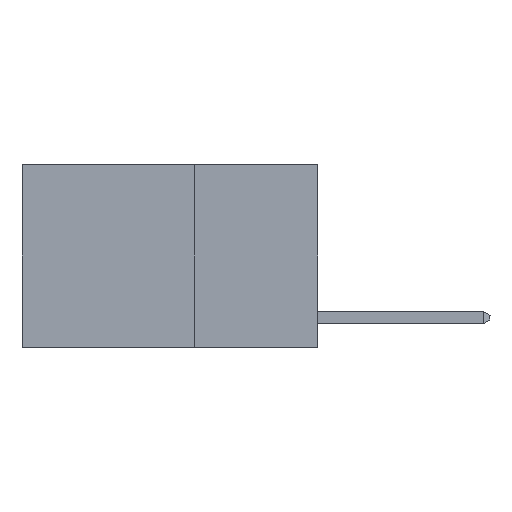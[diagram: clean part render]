
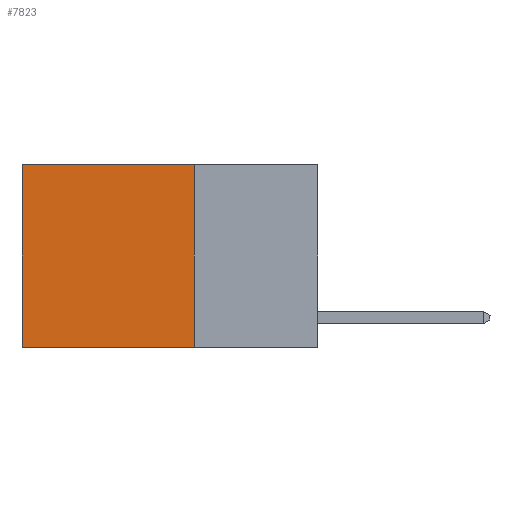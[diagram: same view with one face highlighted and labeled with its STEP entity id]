
A CAD part, left-side view. The second image highlights one B-rep face of the part: STEP entity #7823.
In plain terms, the highlighted planar face has unit normal (-1, 0, 0).
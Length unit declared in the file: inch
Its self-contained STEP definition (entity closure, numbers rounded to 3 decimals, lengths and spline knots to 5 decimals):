
#1244 = LINE ( 'NONE', #2165, #11962 ) ;
#1682 = FACE_OUTER_BOUND ( 'NONE', #6135, .T. ) ;
#2165 = CARTESIAN_POINT ( 'NONE',  ( 0.2625, 0.6, 0. ) ) ;
#3813 = DIRECTION ( 'NONE',  ( 0., 1., 0. ) ) ;
#4150 = CARTESIAN_POINT ( 'NONE',  ( 0.2625, 0.6, 0. ) ) ;
#5239 = CARTESIAN_POINT ( 'NONE',  ( 0.2625, 0.25, 0. ) ) ;
#5268 = VECTOR ( 'NONE', #9627, 39.37008 ) ;
#6135 = EDGE_LOOP ( 'NONE', ( #14003, #6695, #12741, #17709 ) ) ;
#6684 = CARTESIAN_POINT ( 'NONE',  ( 0.2625, 0.25, -0.37 ) ) ;
#6695 = ORIENTED_EDGE ( 'NONE', *, *, #14124, .F. ) ;
#7556 = DIRECTION ( 'NONE',  ( 1., 0., 0. ) ) ;
#7638 = LINE ( 'NONE', #16583, #11419 ) ;
#7823 = ADVANCED_FACE ( 'NONE', ( #1682 ), #10383, .F. ) ;
#8274 = VERTEX_POINT ( 'NONE', #4150 ) ;
#9208 = LINE ( 'NONE', #6684, #17021 ) ;
#9565 = VERTEX_POINT ( 'NONE', #14476 ) ;
#9627 = DIRECTION ( 'NONE',  ( 0., 0., -1. ) ) ;
#9935 = VERTEX_POINT ( 'NONE', #5239 ) ;
#9960 = EDGE_CURVE ( 'NONE', #9935, #8274, #7638, .T. ) ;
#10383 = PLANE ( 'NONE',  #10688 ) ;
#10688 = AXIS2_PLACEMENT_3D ( 'NONE', #15953, #7556, #17321 ) ;
#11043 = CARTESIAN_POINT ( 'NONE',  ( 0.2625, 0.25, 0. ) ) ;
#11203 = EDGE_CURVE ( 'NONE', #9935, #18534, #12937, .T. ) ;
#11419 = VECTOR ( 'NONE', #3813, 39.37008 ) ;
#11962 = VECTOR ( 'NONE', #13748, 39.37008 ) ;
#12741 = ORIENTED_EDGE ( 'NONE', *, *, #11203, .F. ) ;
#12937 = LINE ( 'NONE', #11043, #5268 ) ;
#13748 = DIRECTION ( 'NONE',  ( 0., 0., -1. ) ) ;
#14003 = ORIENTED_EDGE ( 'NONE', *, *, #17116, .T. ) ;
#14081 = CARTESIAN_POINT ( 'NONE',  ( 0.2625, 0.25, -0.37 ) ) ;
#14124 = EDGE_CURVE ( 'NONE', #18534, #9565, #9208, .T. ) ;
#14476 = CARTESIAN_POINT ( 'NONE',  ( 0.2625, 0.6, -0.37 ) ) ;
#15953 = CARTESIAN_POINT ( 'NONE',  ( 0.2625, 0.25, 0. ) ) ;
#16526 = DIRECTION ( 'NONE',  ( 0., 1., 0. ) ) ;
#16583 = CARTESIAN_POINT ( 'NONE',  ( 0.2625, 0.25, 0. ) ) ;
#17021 = VECTOR ( 'NONE', #16526, 39.37008 ) ;
#17116 = EDGE_CURVE ( 'NONE', #8274, #9565, #1244, .T. ) ;
#17321 = DIRECTION ( 'NONE',  ( 0., 0., -1. ) ) ;
#17709 = ORIENTED_EDGE ( 'NONE', *, *, #9960, .T. ) ;
#18534 = VERTEX_POINT ( 'NONE', #14081 ) ;
